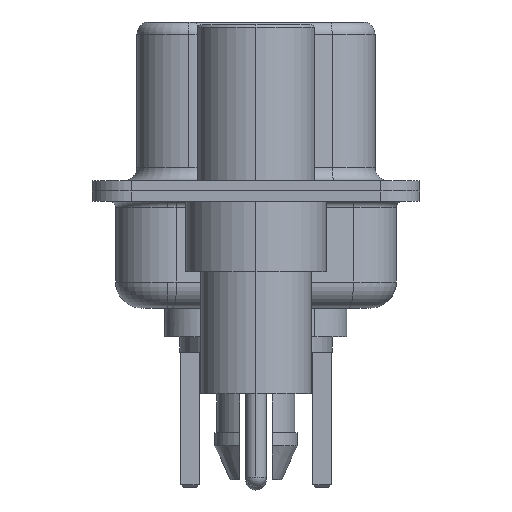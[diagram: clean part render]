
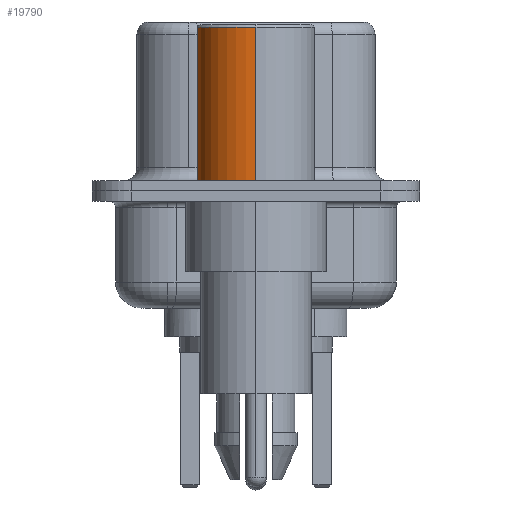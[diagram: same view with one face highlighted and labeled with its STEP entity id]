
A CAD part, left-side view. The second image highlights one B-rep face of the part: STEP entity #19790.
In plain terms, the highlighted cylindrical face has radius 2.25 mm (diameter 4.5 mm), a partial arc.
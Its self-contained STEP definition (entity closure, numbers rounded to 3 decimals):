
#5 = EDGE_CURVE ( 'NONE', #1806, #2879, #19625, .T. ) ;
#55 = CARTESIAN_POINT ( 'NONE',  ( -2.25, 0., 6.3 ) ) ;
#417 = VECTOR ( 'NONE', #1049, 1000. ) ;
#433 = DIRECTION ( 'NONE',  ( 0., 0., 1. ) ) ;
#937 = AXIS2_PLACEMENT_3D ( 'NONE', #5561, #12706, #1265 ) ;
#1049 = DIRECTION ( 'NONE',  ( 0., 0., 1. ) ) ;
#1265 = DIRECTION ( 'NONE',  ( 1., 0., 0. ) ) ;
#1806 = VERTEX_POINT ( 'NONE', #21086 ) ;
#1825 = CARTESIAN_POINT ( 'NONE',  ( 2.25, 0., 0.4 ) ) ;
#2561 = ORIENTED_EDGE ( 'NONE', *, *, #3522, .F. ) ;
#2879 = VERTEX_POINT ( 'NONE', #55 ) ;
#3522 = EDGE_CURVE ( 'NONE', #21327, #1806, #18920, .T. ) ;
#3986 = DIRECTION ( 'NONE',  ( 0., 0., 1. ) ) ;
#4061 = DIRECTION ( 'NONE',  ( 1., 0., 0. ) ) ;
#4669 = EDGE_LOOP ( 'NONE', ( #18562, #8073, #6484, #2561 ) ) ;
#5561 = CARTESIAN_POINT ( 'NONE',  ( 0., 0., 6.3 ) ) ;
#5868 = CARTESIAN_POINT ( 'NONE',  ( 0., 0., 0.4 ) ) ;
#6484 = ORIENTED_EDGE ( 'NONE', *, *, #5, .F. ) ;
#6736 = AXIS2_PLACEMENT_3D ( 'NONE', #14684, #3986, #4061 ) ;
#7381 = CIRCLE ( 'NONE', #11347, 2.25 ) ;
#7690 = DIRECTION ( 'NONE',  ( 1., 0., 0. ) ) ;
#8073 = ORIENTED_EDGE ( 'NONE', *, *, #12137, .T. ) ;
#10914 = CYLINDRICAL_SURFACE ( 'NONE', #6736, 2.25 ) ;
#11347 = AXIS2_PLACEMENT_3D ( 'NONE', #5868, #18293, #7690 ) ;
#11700 = CARTESIAN_POINT ( 'NONE',  ( -2.25, 0., 0.581 ) ) ;
#12137 = EDGE_CURVE ( 'NONE', #14156, #2879, #18786, .T. ) ;
#12706 = DIRECTION ( 'NONE',  ( 0., 0., 1. ) ) ;
#13763 = EDGE_CURVE ( 'NONE', #21327, #14156, #7381, .T. ) ;
#14156 = VERTEX_POINT ( 'NONE', #17429 ) ;
#14684 = CARTESIAN_POINT ( 'NONE',  ( 0., 0., 0.581 ) ) ;
#16180 = FACE_OUTER_BOUND ( 'NONE', #4669, .T. ) ;
#17429 = CARTESIAN_POINT ( 'NONE',  ( -2.25, 0., 0.4 ) ) ;
#18293 = DIRECTION ( 'NONE',  ( 0., 0., 1. ) ) ;
#18371 = VECTOR ( 'NONE', #433, 1000. ) ;
#18562 = ORIENTED_EDGE ( 'NONE', *, *, #13763, .T. ) ;
#18786 = LINE ( 'NONE', #11700, #417 ) ;
#18920 = LINE ( 'NONE', #20932, #18371 ) ;
#19625 = CIRCLE ( 'NONE', #937, 2.25 ) ;
#19790 = ADVANCED_FACE ( 'NONE', ( #16180 ), #10914, .T. ) ;
#20932 = CARTESIAN_POINT ( 'NONE',  ( 2.25, 0., 0.581 ) ) ;
#21086 = CARTESIAN_POINT ( 'NONE',  ( 2.25, 0., 6.3 ) ) ;
#21327 = VERTEX_POINT ( 'NONE', #1825 ) ;
